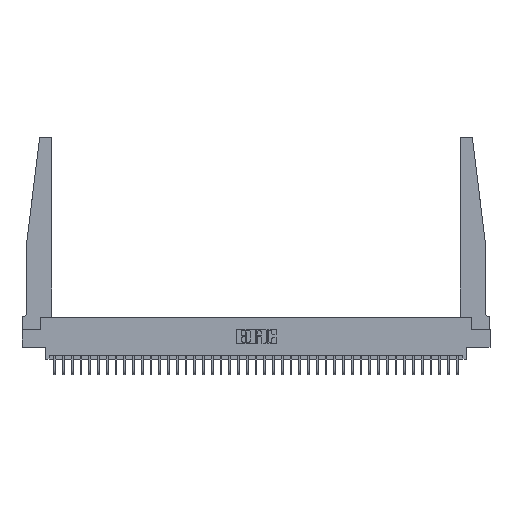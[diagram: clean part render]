
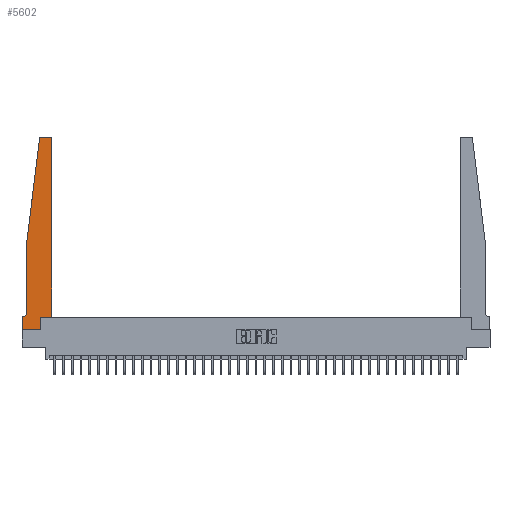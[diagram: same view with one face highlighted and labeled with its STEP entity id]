
A CAD part, top view. The second image highlights one B-rep face of the part: STEP entity #5602.
In plain terms, the highlighted planar face has unit normal (0, 0, 1).
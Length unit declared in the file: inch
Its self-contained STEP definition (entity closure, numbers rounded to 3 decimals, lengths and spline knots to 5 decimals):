
#85 = AXIS2_PLACEMENT_3D ( 'NONE', #6099, #31387, #34272 ) ;
#351 = CIRCLE ( 'NONE', #32107, 0.05 ) ;
#891 = CARTESIAN_POINT ( 'NONE',  ( 0.395, 2.75, 0.37 ) ) ;
#1252 = EDGE_CURVE ( 'NONE', #17424, #7185, #18565, .T. ) ;
#1721 = VECTOR ( 'NONE', #25944, 39.37008 ) ;
#1824 = EDGE_CURVE ( 'NONE', #22871, #9292, #33696, .T. ) ;
#2098 = EDGE_CURVE ( 'NONE', #11227, #23979, #36345, .T. ) ;
#2631 = DIRECTION ( 'NONE',  ( 0., -1., 0. ) ) ;
#2750 = CARTESIAN_POINT ( 'NONE',  ( 0.065, 1.25, 0.37 ) ) ;
#2935 = CARTESIAN_POINT ( 'NONE',  ( 0.425, 0.18, 0.37 ) ) ;
#3080 = VECTOR ( 'NONE', #15166, 39.37008 ) ;
#3416 = LINE ( 'NONE', #30052, #19414 ) ;
#4190 = EDGE_CURVE ( 'NONE', #30639, #4906, #25095, .T. ) ;
#4195 = CARTESIAN_POINT ( 'NONE',  ( 0.425, 2.72, 0.37 ) ) ;
#4906 = VERTEX_POINT ( 'NONE', #14372 ) ;
#5017 = CARTESIAN_POINT ( 'NONE',  ( 0.2605, 0., 0.37 ) ) ;
#5593 = EDGE_CURVE ( 'NONE', #23979, #28527, #8682, .T. ) ;
#5602 = ADVANCED_FACE ( 'NONE', ( #11381 ), #28104, .T. ) ;
#5993 = CIRCLE ( 'NONE', #85, 0.03 ) ;
#6099 = CARTESIAN_POINT ( 'NONE',  ( 0.395, 2.72, 0.37 ) ) ;
#6272 = CARTESIAN_POINT ( 'NONE',  ( 0.065, 1.25, 0.37 ) ) ;
#6340 = CARTESIAN_POINT ( 'NONE',  ( 0.2605, 0.18, 0.37 ) ) ;
#6941 = EDGE_CURVE ( 'NONE', #28527, #17424, #22715, .T. ) ;
#7185 = VERTEX_POINT ( 'NONE', #4195 ) ;
#7745 = VERTEX_POINT ( 'NONE', #28346 ) ;
#7754 = CARTESIAN_POINT ( 'NONE',  ( 0.425, 0.18, 0.37 ) ) ;
#7986 = LINE ( 'NONE', #34618, #3080 ) ;
#8304 = AXIS2_PLACEMENT_3D ( 'NONE', #25250, #28258, #16986 ) ;
#8655 = DIRECTION ( 'NONE',  ( 0., 1., 0. ) ) ;
#8682 = LINE ( 'NONE', #6340, #17506 ) ;
#9292 = VERTEX_POINT ( 'NONE', #25272 ) ;
#9670 = AXIS2_PLACEMENT_3D ( 'NONE', #13931, #14043, #34636 ) ;
#10228 = EDGE_CURVE ( 'NONE', #9292, #7745, #35224, .T. ) ;
#10238 = VECTOR ( 'NONE', #2631, 39.37008 ) ;
#10275 = DIRECTION ( 'NONE',  ( 1., 0., 0. ) ) ;
#10480 = CARTESIAN_POINT ( 'NONE',  ( 0.015, 0.2375, 0.37 ) ) ;
#10580 = ORIENTED_EDGE ( 'NONE', *, *, #26890, .T. ) ;
#11022 = EDGE_LOOP ( 'NONE', ( #30379, #24827, #29639, #10580, #17925, #35366, #33797, #21531, #30286, #19794, #13989, #17965 ) ) ;
#11227 = VERTEX_POINT ( 'NONE', #21371 ) ;
#11308 = VECTOR ( 'NONE', #22930, 39.37008 ) ;
#11381 = FACE_OUTER_BOUND ( 'NONE', #11022, .T. ) ;
#13007 = EDGE_CURVE ( 'NONE', #4906, #11227, #7986, .T. ) ;
#13419 = DIRECTION ( 'NONE',  ( 0., 0., -1. ) ) ;
#13500 = CARTESIAN_POINT ( 'NONE',  ( 0.2605, 0.18, 0.37 ) ) ;
#13931 = CARTESIAN_POINT ( 'NONE',  ( 0., 0.1875, 0.37 ) ) ;
#13989 = ORIENTED_EDGE ( 'NONE', *, *, #1252, .T. ) ;
#14043 = DIRECTION ( 'NONE',  ( 0., 0., 1. ) ) ;
#14372 = CARTESIAN_POINT ( 'NONE',  ( 0., 0.1875, 0.37 ) ) ;
#15069 = DIRECTION ( 'NONE',  ( 0., 1., 0. ) ) ;
#15166 = DIRECTION ( 'NONE',  ( 0., -1., 0. ) ) ;
#16589 = DIRECTION ( 'NONE',  ( -1., 0., 0. ) ) ;
#16986 = DIRECTION ( 'NONE',  ( 1., 0., 0. ) ) ;
#17424 = VERTEX_POINT ( 'NONE', #31289 ) ;
#17506 = VECTOR ( 'NONE', #15069, 39.37008 ) ;
#17925 = ORIENTED_EDGE ( 'NONE', *, *, #34264, .T. ) ;
#17965 = ORIENTED_EDGE ( 'NONE', *, *, #35714, .T. ) ;
#18497 = VECTOR ( 'NONE', #16589, 39.37008 ) ;
#18565 = LINE ( 'NONE', #2935, #19473 ) ;
#19414 = VECTOR ( 'NONE', #27475, 39.37008 ) ;
#19473 = VECTOR ( 'NONE', #8655, 39.37008 ) ;
#19794 = ORIENTED_EDGE ( 'NONE', *, *, #6941, .T. ) ;
#20276 = CARTESIAN_POINT ( 'NONE',  ( 0., 0., 0.37 ) ) ;
#21371 = CARTESIAN_POINT ( 'NONE',  ( 0., 0., 0.37 ) ) ;
#21531 = ORIENTED_EDGE ( 'NONE', *, *, #2098, .T. ) ;
#22715 = LINE ( 'NONE', #7754, #23591 ) ;
#22871 = VERTEX_POINT ( 'NONE', #31117 ) ;
#22930 = DIRECTION ( 'NONE',  ( -0.122, -0.992, 0. ) ) ;
#23591 = VECTOR ( 'NONE', #10275, 39.37008 ) ;
#23600 = VERTEX_POINT ( 'NONE', #26204 ) ;
#23979 = VERTEX_POINT ( 'NONE', #5017 ) ;
#24711 = CARTESIAN_POINT ( 'NONE',  ( 0.015, 0.1875, 0.37 ) ) ;
#24827 = ORIENTED_EDGE ( 'NONE', *, *, #1824, .T. ) ;
#24899 = DIRECTION ( 'NONE',  ( -1., 0., 0. ) ) ;
#25095 = LINE ( 'NONE', #28213, #18497 ) ;
#25231 = LINE ( 'NONE', #2750, #10238 ) ;
#25250 = CARTESIAN_POINT ( 'NONE',  ( 0.27653, 2.72, 0.37 ) ) ;
#25272 = CARTESIAN_POINT ( 'NONE',  ( 0.24675, 2.72367, 0.37 ) ) ;
#25944 = DIRECTION ( 'NONE',  ( 1., 0., 0. ) ) ;
#26204 = CARTESIAN_POINT ( 'NONE',  ( 0.065, 0.2375, 0.37 ) ) ;
#26890 = EDGE_CURVE ( 'NONE', #7745, #23600, #25231, .T. ) ;
#27475 = DIRECTION ( 'NONE',  ( -1., 0., 0. ) ) ;
#28104 = PLANE ( 'NONE',  #9670 ) ;
#28213 = CARTESIAN_POINT ( 'NONE',  ( 0.065, 0.1875, 0.37 ) ) ;
#28258 = DIRECTION ( 'NONE',  ( 0., 0., 1. ) ) ;
#28346 = CARTESIAN_POINT ( 'NONE',  ( 0.065, 1.25, 0.37 ) ) ;
#28413 = EDGE_CURVE ( 'NONE', #33965, #22871, #3416, .T. ) ;
#28527 = VERTEX_POINT ( 'NONE', #13500 ) ;
#29639 = ORIENTED_EDGE ( 'NONE', *, *, #10228, .T. ) ;
#30052 = CARTESIAN_POINT ( 'NONE',  ( 0.25, 2.75, 0.37 ) ) ;
#30286 = ORIENTED_EDGE ( 'NONE', *, *, #5593, .T. ) ;
#30379 = ORIENTED_EDGE ( 'NONE', *, *, #28413, .T. ) ;
#30639 = VERTEX_POINT ( 'NONE', #24711 ) ;
#31117 = CARTESIAN_POINT ( 'NONE',  ( 0.27653, 2.75, 0.37 ) ) ;
#31289 = CARTESIAN_POINT ( 'NONE',  ( 0.425, 0.18, 0.37 ) ) ;
#31387 = DIRECTION ( 'NONE',  ( 0., 0., 1. ) ) ;
#32107 = AXIS2_PLACEMENT_3D ( 'NONE', #10480, #13419, #24899 ) ;
#33696 = CIRCLE ( 'NONE', #8304, 0.03 ) ;
#33797 = ORIENTED_EDGE ( 'NONE', *, *, #13007, .T. ) ;
#33965 = VERTEX_POINT ( 'NONE', #891 ) ;
#34264 = EDGE_CURVE ( 'NONE', #23600, #30639, #351, .T. ) ;
#34272 = DIRECTION ( 'NONE',  ( 1., 0., 0. ) ) ;
#34618 = CARTESIAN_POINT ( 'NONE',  ( 0., 0., 0.37 ) ) ;
#34636 = DIRECTION ( 'NONE',  ( 1., 0., 0. ) ) ;
#35224 = LINE ( 'NONE', #6272, #11308 ) ;
#35366 = ORIENTED_EDGE ( 'NONE', *, *, #4190, .T. ) ;
#35714 = EDGE_CURVE ( 'NONE', #7185, #33965, #5993, .T. ) ;
#36345 = LINE ( 'NONE', #20276, #1721 ) ;
